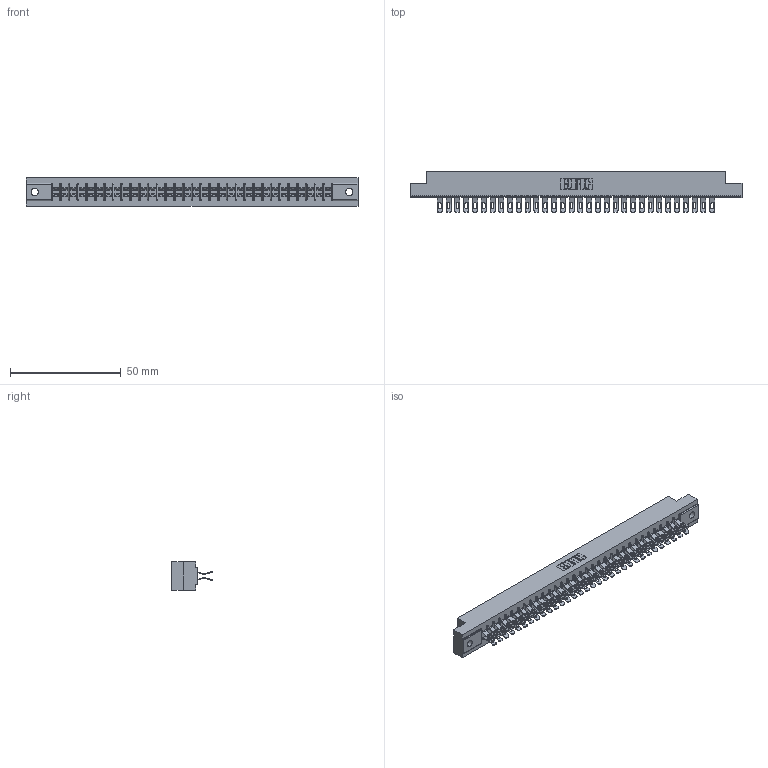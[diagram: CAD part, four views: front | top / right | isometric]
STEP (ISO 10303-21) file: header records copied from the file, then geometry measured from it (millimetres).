
FILE_DESCRIPTION (( 'STEP AP203' ), '1' );
FILE_NAME ('315-064-555-202.STEP', '2019-09-10T20:36:27', ( '' ), ( '' ), 'SwSTEP 2.0', 'SolidWorks 2016', '' );
FILE_SCHEMA (( 'CONFIG_CONTROL_DESIGN' ));
Length unit declared in the file: inch
Products named in the file (3): 305 Part_.128 Dia; 315-064-555-202; 305-290-001_555
Assembly tree (65 placements, depth 2):
  315-064-555-202
    305 Part_.128 Dia
    305-290-001_555  x64
Bounding box: 149.81 x 18.41 x 12.7 mm (x, y, z)
Volume: 15724.3 mm3; surface area: 20701.3 mm2
Topology: 65 solids, 65 shells, 4340 faces, 12956 edges, 8464 vertices
Faces by surface type: plane 2116, cylinder 2096, sphere 128
Entity records: 36491 total; most frequent: CARTESIAN_POINT 6056, ORIENTED_EDGE 6000, DIRECTION 5860, EDGE_CURVE 3000, LINE 2396, VECTOR 2396, VERTEX_POINT 1912, AXIS2_PLACEMENT_3D 1732
